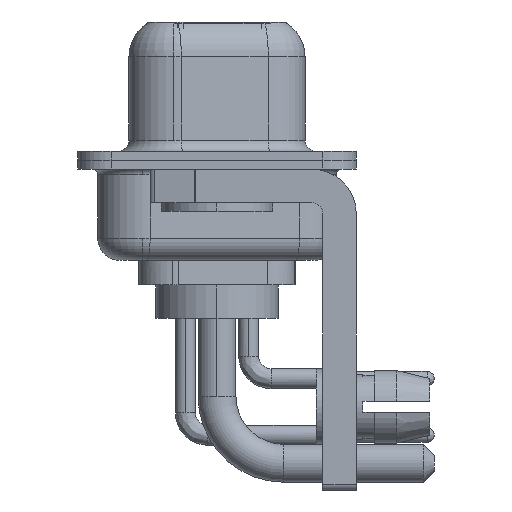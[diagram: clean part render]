
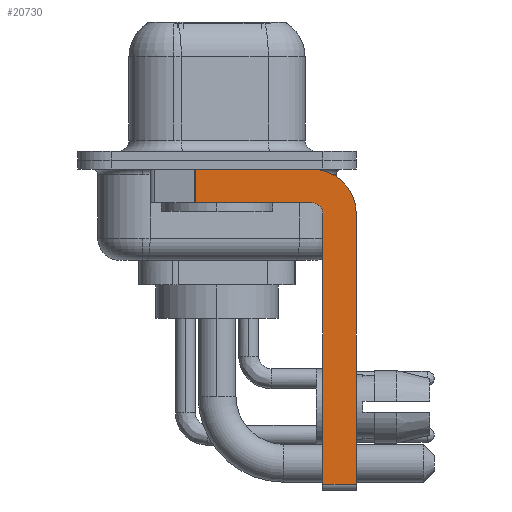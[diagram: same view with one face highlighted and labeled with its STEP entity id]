
A CAD part, left-side view. The second image highlights one B-rep face of the part: STEP entity #20730.
In plain terms, the highlighted planar face has unit normal (-1, 0, 0).
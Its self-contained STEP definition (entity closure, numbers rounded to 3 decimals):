
#192 = CARTESIAN_POINT ( 'NONE',  ( -2.9, -4.25, -14.55 ) ) ;
#275 = ORIENTED_EDGE ( 'NONE', *, *, #13390, .T. ) ;
#708 = EDGE_CURVE ( 'NONE', #15712, #11277, #21938, .T. ) ;
#1566 = DIRECTION ( 'NONE',  ( 0., 0., 1. ) ) ;
#1679 = VECTOR ( 'NONE', #1811, 1000. ) ;
#1811 = DIRECTION ( 'NONE',  ( 0., -1., 0. ) ) ;
#2014 = CARTESIAN_POINT ( 'NONE',  ( -2.9, -4.25, -0.4 ) ) ;
#2663 = DIRECTION ( 'NONE',  ( 0., 0., -1. ) ) ;
#3023 = EDGE_CURVE ( 'NONE', #9309, #11753, #17670, .T. ) ;
#3092 = AXIS2_PLACEMENT_3D ( 'NONE', #17721, #7418, #3556 ) ;
#3386 = CARTESIAN_POINT ( 'NONE',  ( -2.9, -4.75, -14.55 ) ) ;
#3556 = DIRECTION ( 'NONE',  ( 0., 0., -1. ) ) ;
#3631 = CARTESIAN_POINT ( 'NONE',  ( -2.9, 3., -0.4 ) ) ;
#3658 = ORIENTED_EDGE ( 'NONE', *, *, #12491, .F. ) ;
#4049 = ORIENTED_EDGE ( 'NONE', *, *, #12414, .F. ) ;
#4539 = LINE ( 'NONE', #16966, #9226 ) ;
#4756 = LINE ( 'NONE', #25006, #25345 ) ;
#5043 = VECTOR ( 'NONE', #21145, 1000. ) ;
#7005 = LINE ( 'NONE', #16652, #5043 ) ;
#7122 = ORIENTED_EDGE ( 'NONE', *, *, #708, .F. ) ;
#7418 = DIRECTION ( 'NONE',  ( 1., 0., 0. ) ) ;
#7694 = LINE ( 'NONE', #9934, #9129 ) ;
#8153 = ORIENTED_EDGE ( 'NONE', *, *, #3023, .F. ) ;
#8744 = ORIENTED_EDGE ( 'NONE', *, *, #11408, .F. ) ;
#9129 = VECTOR ( 'NONE', #1566, 1000. ) ;
#9226 = VECTOR ( 'NONE', #2663, 1000. ) ;
#9272 = CARTESIAN_POINT ( 'NONE',  ( -2.9, -6.25, -14.55 ) ) ;
#9309 = VERTEX_POINT ( 'NONE', #15911 ) ;
#9772 = DIRECTION ( 'NONE',  ( 0., 0., -1. ) ) ;
#9934 = CARTESIAN_POINT ( 'NONE',  ( -2.9, -4.75, -14.8 ) ) ;
#10220 = VERTEX_POINT ( 'NONE', #9272 ) ;
#10338 = VERTEX_POINT ( 'NONE', #22083 ) ;
#10547 = AXIS2_PLACEMENT_3D ( 'NONE', #18920, #17058, #23141 ) ;
#11037 = EDGE_CURVE ( 'NONE', #9309, #10338, #4539, .T. ) ;
#11277 = VERTEX_POINT ( 'NONE', #13346 ) ;
#11408 = EDGE_CURVE ( 'NONE', #11753, #16051, #15151, .T. ) ;
#11753 = VERTEX_POINT ( 'NONE', #2014 ) ;
#12414 = EDGE_CURVE ( 'NONE', #16051, #10220, #7005, .T. ) ;
#12491 = EDGE_CURVE ( 'NONE', #11277, #10338, #4756, .T. ) ;
#13346 = CARTESIAN_POINT ( 'NONE',  ( -2.9, -4.25, -1.9 ) ) ;
#13390 = EDGE_CURVE ( 'NONE', #16333, #10220, #16502, .T. ) ;
#15151 = CIRCLE ( 'NONE', #18519, 2. ) ;
#15712 = VERTEX_POINT ( 'NONE', #18963 ) ;
#15911 = CARTESIAN_POINT ( 'NONE',  ( -2.9, 0.978, -0.4 ) ) ;
#16051 = VERTEX_POINT ( 'NONE', #22338 ) ;
#16333 = VERTEX_POINT ( 'NONE', #3386 ) ;
#16502 = LINE ( 'NONE', #192, #1679 ) ;
#16652 = CARTESIAN_POINT ( 'NONE',  ( -2.9, -6.25, -2.4 ) ) ;
#16966 = CARTESIAN_POINT ( 'NONE',  ( -2.9, 0.978, -1.9 ) ) ;
#17058 = DIRECTION ( 'NONE',  ( -1., 0., 0. ) ) ;
#17401 = DIRECTION ( 'NONE',  ( 0., -1., 0. ) ) ;
#17670 = LINE ( 'NONE', #3631, #25952 ) ;
#17721 = CARTESIAN_POINT ( 'NONE',  ( -2.9, -4.25, -2.4 ) ) ;
#17927 = ORIENTED_EDGE ( 'NONE', *, *, #11037, .T. ) ;
#18519 = AXIS2_PLACEMENT_3D ( 'NONE', #26164, #26035, #9772 ) ;
#18920 = CARTESIAN_POINT ( 'NONE',  ( -2.9, -4.25, -2.4 ) ) ;
#18963 = CARTESIAN_POINT ( 'NONE',  ( -2.9, -4.75, -2.4 ) ) ;
#19828 = PLANE ( 'NONE',  #3092 ) ;
#20562 = ORIENTED_EDGE ( 'NONE', *, *, #22975, .F. ) ;
#20730 = ADVANCED_FACE ( 'NONE', ( #21823 ), #19828, .F. ) ;
#21145 = DIRECTION ( 'NONE',  ( 0., 0., -1. ) ) ;
#21823 = FACE_OUTER_BOUND ( 'NONE', #22526, .T. ) ;
#21938 = CIRCLE ( 'NONE', #10547, 0.5 ) ;
#22083 = CARTESIAN_POINT ( 'NONE',  ( -2.9, 0.978, -1.9 ) ) ;
#22338 = CARTESIAN_POINT ( 'NONE',  ( -2.9, -6.25, -2.4 ) ) ;
#22526 = EDGE_LOOP ( 'NONE', ( #8153, #17927, #3658, #7122, #20562, #275, #4049, #8744 ) ) ;
#22975 = EDGE_CURVE ( 'NONE', #16333, #15712, #7694, .T. ) ;
#23141 = DIRECTION ( 'NONE',  ( 0., 0., 1. ) ) ;
#25006 = CARTESIAN_POINT ( 'NONE',  ( -2.9, -4.25, -1.9 ) ) ;
#25345 = VECTOR ( 'NONE', #25795, 1000. ) ;
#25795 = DIRECTION ( 'NONE',  ( 0., 1., 0. ) ) ;
#25952 = VECTOR ( 'NONE', #17401, 1000. ) ;
#26035 = DIRECTION ( 'NONE',  ( 1., 0., 0. ) ) ;
#26164 = CARTESIAN_POINT ( 'NONE',  ( -2.9, -4.25, -2.4 ) ) ;
